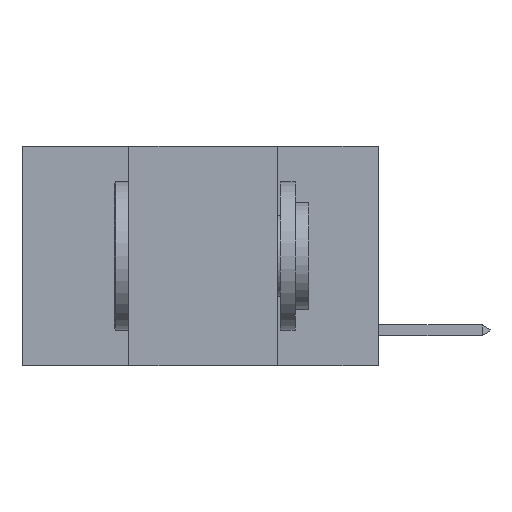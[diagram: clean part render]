
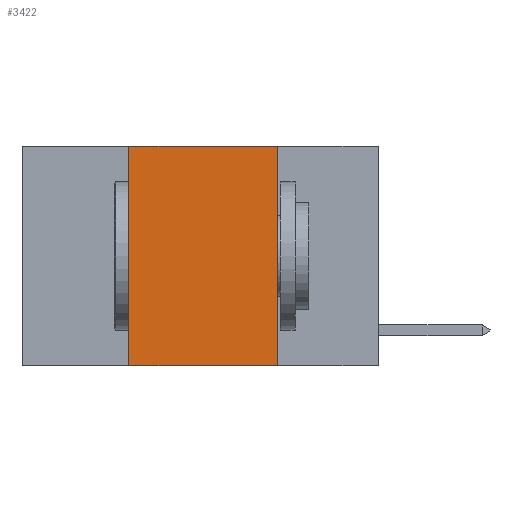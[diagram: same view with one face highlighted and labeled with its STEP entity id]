
A CAD part, left-side view. The second image highlights one B-rep face of the part: STEP entity #3422.
In plain terms, the highlighted planar face has unit normal (-1, 0, 0).
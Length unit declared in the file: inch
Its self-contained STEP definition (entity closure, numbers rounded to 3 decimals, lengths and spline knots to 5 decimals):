
#246 = LINE ( 'NONE', #13689, #13828 ) ;
#1370 = PLANE ( 'NONE',  #17802 ) ;
#1507 = EDGE_CURVE ( 'NONE', #11342, #1655, #6923, .T. ) ;
#1655 = VERTEX_POINT ( 'NONE', #4673 ) ;
#2994 = DIRECTION ( 'NONE',  ( 0., 0., -1. ) ) ;
#3422 = ADVANCED_FACE ( 'NONE', ( #8923 ), #1370, .F. ) ;
#4002 = CARTESIAN_POINT ( 'NONE',  ( 0., 0.6, 0. ) ) ;
#4673 = CARTESIAN_POINT ( 'NONE',  ( 0., 0.17, 0. ) ) ;
#4753 = ORIENTED_EDGE ( 'NONE', *, *, #15509, .F. ) ;
#4829 = VECTOR ( 'NONE', #17926, 39.37008 ) ;
#5820 = DIRECTION ( 'NONE',  ( 1., 0., 0. ) ) ;
#6118 = LINE ( 'NONE', #12029, #4829 ) ;
#6598 = VERTEX_POINT ( 'NONE', #9865 ) ;
#6923 = LINE ( 'NONE', #4002, #8086 ) ;
#7036 = ORIENTED_EDGE ( 'NONE', *, *, #16067, .F. ) ;
#7369 = VERTEX_POINT ( 'NONE', #12302 ) ;
#7665 = CARTESIAN_POINT ( 'NONE',  ( 0., 0.6, -0.37 ) ) ;
#8086 = VECTOR ( 'NONE', #18827, 39.37008 ) ;
#8923 = FACE_OUTER_BOUND ( 'NONE', #13418, .T. ) ;
#9865 = CARTESIAN_POINT ( 'NONE',  ( 0., 0.42, -0.37 ) ) ;
#10769 = DIRECTION ( 'NONE',  ( 0., -1., 0. ) ) ;
#11342 = VERTEX_POINT ( 'NONE', #11658 ) ;
#11658 = CARTESIAN_POINT ( 'NONE',  ( 0., 0.42, 0. ) ) ;
#11850 = ORIENTED_EDGE ( 'NONE', *, *, #1507, .F. ) ;
#12029 = CARTESIAN_POINT ( 'NONE',  ( 0., 0.17, 0. ) ) ;
#12302 = CARTESIAN_POINT ( 'NONE',  ( 0., 0.17, -0.37 ) ) ;
#13418 = EDGE_LOOP ( 'NONE', ( #7036, #11850, #4753, #17484 ) ) ;
#13446 = CARTESIAN_POINT ( 'NONE',  ( 0., 0.6, 0. ) ) ;
#13689 = CARTESIAN_POINT ( 'NONE',  ( 0., 0.42, 0. ) ) ;
#13828 = VECTOR ( 'NONE', #18137, 39.37008 ) ;
#14587 = EDGE_CURVE ( 'NONE', #6598, #7369, #15126, .T. ) ;
#15126 = LINE ( 'NONE', #7665, #16599 ) ;
#15509 = EDGE_CURVE ( 'NONE', #6598, #11342, #246, .T. ) ;
#16067 = EDGE_CURVE ( 'NONE', #1655, #7369, #6118, .T. ) ;
#16599 = VECTOR ( 'NONE', #10769, 39.37008 ) ;
#17484 = ORIENTED_EDGE ( 'NONE', *, *, #14587, .T. ) ;
#17802 = AXIS2_PLACEMENT_3D ( 'NONE', #13446, #5820, #2994 ) ;
#17926 = DIRECTION ( 'NONE',  ( 0., 0., -1. ) ) ;
#18137 = DIRECTION ( 'NONE',  ( 0., 0., 1. ) ) ;
#18827 = DIRECTION ( 'NONE',  ( 0., -1., 0. ) ) ;
